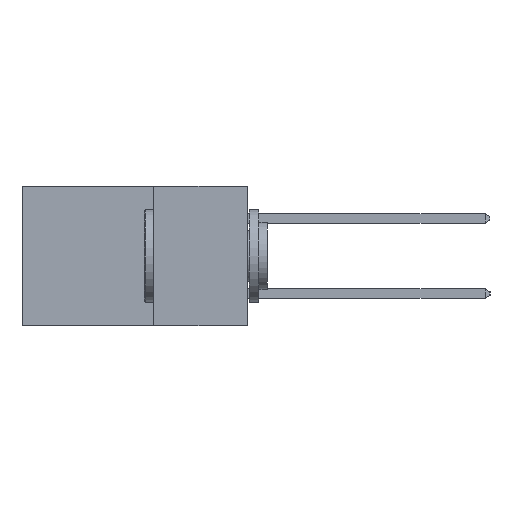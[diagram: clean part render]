
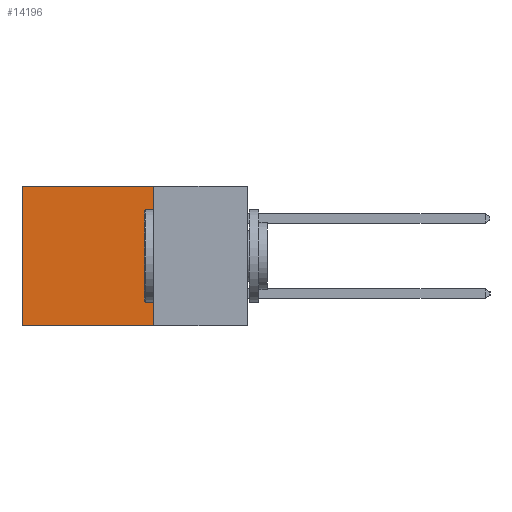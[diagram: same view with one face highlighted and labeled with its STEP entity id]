
A CAD part, left-side view. The second image highlights one B-rep face of the part: STEP entity #14196.
In plain terms, the highlighted planar face has unit normal (-1, 0, 0).
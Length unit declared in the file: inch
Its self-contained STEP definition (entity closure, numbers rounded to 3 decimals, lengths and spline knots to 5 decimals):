
#1215 = EDGE_CURVE ( 'NONE', #3195, #24625, #24383, .T. ) ;
#1772 = PLANE ( 'NONE',  #10464 ) ;
#2507 = CARTESIAN_POINT ( 'NONE',  ( 0.2615, 0.6, -0.37 ) ) ;
#3195 = VERTEX_POINT ( 'NONE', #23059 ) ;
#3456 = DIRECTION ( 'NONE',  ( 0., 1., 0. ) ) ;
#3687 = DIRECTION ( 'NONE',  ( 0., 0., -1. ) ) ;
#5003 = CARTESIAN_POINT ( 'NONE',  ( 0.2615, 0.25, -0.37 ) ) ;
#6077 = CARTESIAN_POINT ( 'NONE',  ( 0.2615, 0.6, 0. ) ) ;
#6322 = ORIENTED_EDGE ( 'NONE', *, *, #15892, .F. ) ;
#6500 = EDGE_CURVE ( 'NONE', #24625, #24057, #16993, .T. ) ;
#7771 = VECTOR ( 'NONE', #9931, 39.37008 ) ;
#8019 = DIRECTION ( 'NONE',  ( 0., 1., 0. ) ) ;
#9931 = DIRECTION ( 'NONE',  ( 0., 0., -1. ) ) ;
#10464 = AXIS2_PLACEMENT_3D ( 'NONE', #24519, #20742, #3687 ) ;
#11645 = FACE_OUTER_BOUND ( 'NONE', #12338, .T. ) ;
#12081 = DIRECTION ( 'NONE',  ( 0., 0., -1. ) ) ;
#12338 = EDGE_LOOP ( 'NONE', ( #13340, #6322, #23599, #14615 ) ) ;
#13340 = ORIENTED_EDGE ( 'NONE', *, *, #6500, .T. ) ;
#13698 = EDGE_CURVE ( 'NONE', #3195, #16888, #22258, .T. ) ;
#13927 = LINE ( 'NONE', #23147, #23340 ) ;
#14196 = ADVANCED_FACE ( 'NONE', ( #11645 ), #1772, .F. ) ;
#14366 = VECTOR ( 'NONE', #3456, 39.37008 ) ;
#14615 = ORIENTED_EDGE ( 'NONE', *, *, #1215, .T. ) ;
#15892 = EDGE_CURVE ( 'NONE', #16888, #24057, #13927, .T. ) ;
#16410 = VECTOR ( 'NONE', #12081, 39.37008 ) ;
#16888 = VERTEX_POINT ( 'NONE', #5003 ) ;
#16993 = LINE ( 'NONE', #2507, #16410 ) ;
#17489 = CARTESIAN_POINT ( 'NONE',  ( 0.2615, 0.25, -0.37 ) ) ;
#17968 = CARTESIAN_POINT ( 'NONE',  ( 0.2615, 0.6, -0.37 ) ) ;
#20742 = DIRECTION ( 'NONE',  ( 1., 0., 0. ) ) ;
#22258 = LINE ( 'NONE', #17489, #7771 ) ;
#23059 = CARTESIAN_POINT ( 'NONE',  ( 0.2615, 0.25, 0. ) ) ;
#23147 = CARTESIAN_POINT ( 'NONE',  ( 0.2615, 0.25, -0.37 ) ) ;
#23340 = VECTOR ( 'NONE', #8019, 39.37008 ) ;
#23599 = ORIENTED_EDGE ( 'NONE', *, *, #13698, .F. ) ;
#23605 = CARTESIAN_POINT ( 'NONE',  ( 0.2615, 0.25, 0. ) ) ;
#24057 = VERTEX_POINT ( 'NONE', #17968 ) ;
#24383 = LINE ( 'NONE', #23605, #14366 ) ;
#24519 = CARTESIAN_POINT ( 'NONE',  ( 0.2615, 0.25, -0.37 ) ) ;
#24625 = VERTEX_POINT ( 'NONE', #6077 ) ;
